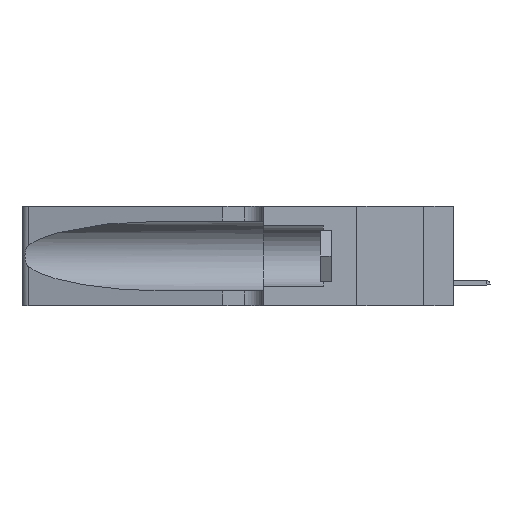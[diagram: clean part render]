
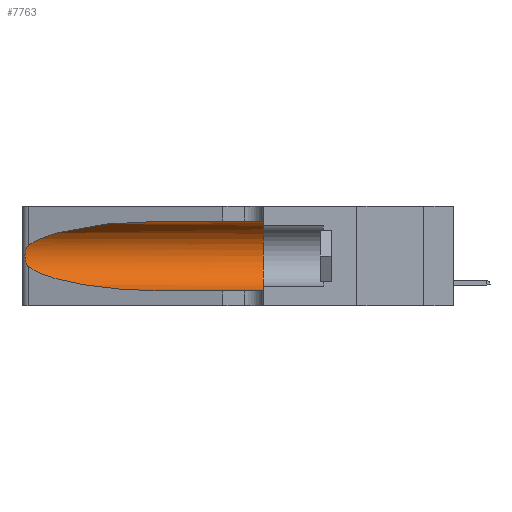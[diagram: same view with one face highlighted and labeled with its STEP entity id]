
A CAD part, left-side view. The second image highlights one B-rep face of the part: STEP entity #7763.
In plain terms, the highlighted cylindrical face has radius 3.308 mm (diameter 6.617 mm), a partial arc.
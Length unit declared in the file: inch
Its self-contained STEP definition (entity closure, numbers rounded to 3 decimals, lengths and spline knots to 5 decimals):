
#553 = CARTESIAN_POINT ( 'NONE',  ( 0.2373, 1.15595, 0.08982 ) ) ;
#1433 = VERTEX_POINT ( 'NONE', #5985 ) ;
#1889 = LINE ( 'NONE', #8013, #12411 ) ;
#2998 = CARTESIAN_POINT ( 'NONE',  ( 0.1305, 1.61858, 0.185 ) ) ;
#3121 = EDGE_CURVE ( 'NONE', #13543, #18669, #11058, .T. ) ;
#3147 = AXIS2_PLACEMENT_3D ( 'NONE', #6868, #18050, #10074 ) ;
#3162 = ORIENTED_EDGE ( 'NONE', *, *, #3121, .T. ) ;
#3216 = DIRECTION ( 'NONE',  ( 0., 0., -1. ) ) ;
#3707 = VERTEX_POINT ( 'NONE', #13667 ) ;
#4069 = CARTESIAN_POINT ( 'NONE',  ( 0.25854, 1.2359, 0.20912 ) ) ;
#5098 = B_SPLINE_CURVE_WITH_KNOTS ( 'NONE', 3,
 ( #20478, #20588, #10875, #18629, #4069, #10568, #12259, #18740, #16200, #16524, #8134, #11315, #17808, #18129 ),
 .UNSPECIFIED., .F., .F.,
 ( 4, 2, 2, 2, 2, 2, 4 ),
 ( 0., 0.00027, 0.00053, 0.00107, 0.0016, 0.00187, 0.00214 ),
 .UNSPECIFIED. ) ;
#5554 = CARTESIAN_POINT ( 'NONE',  ( 0.2373, 1.15595, 0.28018 ) ) ;
#5985 = CARTESIAN_POINT ( 'NONE',  ( 0.1305, 0.72297, 0.05475 ) ) ;
#6702 =( BOUNDED_CURVE ( )  B_SPLINE_CURVE ( 3, ( #13577, #553, #7199, #13686 ),
 .UNSPECIFIED., .F., .T. ) 
 B_SPLINE_CURVE_WITH_KNOTS ( ( 4, 4 ),
 ( 3.44316, 4.71239 ),
 .UNSPECIFIED. ) 
 CURVE ( )  GEOMETRIC_REPRESENTATION_ITEM ( )  RATIONAL_B_SPLINE_CURVE ( ( 1., 0.87, 0.87, 1. ) ) 
 REPRESENTATION_ITEM ( '' )  );
#6868 = CARTESIAN_POINT ( 'NONE',  ( 0.1305, 0.35, 0.185 ) ) ;
#7199 = CARTESIAN_POINT ( 'NONE',  ( 0.18966, 0.96281, 0.05475 ) ) ;
#7763 = ADVANCED_FACE ( 'NONE', ( #19625 ), #21017, .F. ) ;
#7794 = CARTESIAN_POINT ( 'NONE',  ( 0.1305, 1.61858, 0.31525 ) ) ;
#8013 = CARTESIAN_POINT ( 'NONE',  ( 0.1305, 1.61858, 0.05475 ) ) ;
#8134 = CARTESIAN_POINT ( 'NONE',  ( 0.25789, 1.23486, 0.15765 ) ) ;
#8591 = CARTESIAN_POINT ( 'NONE',  ( 0.1305, 0.35, 0.05475 ) ) ;
#9080 = EDGE_CURVE ( 'NONE', #18669, #17951, #5098, .T. ) ;
#9188 = CARTESIAN_POINT ( 'NONE',  ( 0.1305, 0.72297, 0.31525 ) ) ;
#10074 = DIRECTION ( 'NONE',  ( 0., 0., 1. ) ) ;
#10568 = CARTESIAN_POINT ( 'NONE',  ( 0.26018, 1.23835, 0.19895 ) ) ;
#10875 = CARTESIAN_POINT ( 'NONE',  ( 0.25639, 1.23184, 0.21858 ) ) ;
#11058 =( BOUNDED_CURVE ( )  B_SPLINE_CURVE ( 3, ( #15146, #20172, #5554, #12067 ),
 .UNSPECIFIED., .F., .T. ) 
 B_SPLINE_CURVE_WITH_KNOTS ( ( 4, 4 ),
 ( 1.5708, 2.84003 ),
 .UNSPECIFIED. ) 
 CURVE ( )  GEOMETRIC_REPRESENTATION_ITEM ( )  RATIONAL_B_SPLINE_CURVE ( ( 1., 0.87, 0.87, 1. ) ) 
 REPRESENTATION_ITEM ( '' )  );
#11315 = CARTESIAN_POINT ( 'NONE',  ( 0.25639, 1.23186, 0.15144 ) ) ;
#12067 = CARTESIAN_POINT ( 'NONE',  ( 0.25487, 1.22718, 0.22369 ) ) ;
#12256 = VECTOR ( 'NONE', #14303, 39.37008 ) ;
#12259 = CARTESIAN_POINT ( 'NONE',  ( 0.26075, 1.23896, 0.19203 ) ) ;
#12411 = VECTOR ( 'NONE', #16303, 39.37008 ) ;
#12804 = DIRECTION ( 'NONE',  ( 0., -1., 0. ) ) ;
#12899 = EDGE_CURVE ( 'NONE', #1433, #13908, #1889, .T. ) ;
#12971 = ORIENTED_EDGE ( 'NONE', *, *, #17817, .T. ) ;
#13543 = VERTEX_POINT ( 'NONE', #9188 ) ;
#13577 = CARTESIAN_POINT ( 'NONE',  ( 0.25487, 1.22718, 0.14631 ) ) ;
#13667 = CARTESIAN_POINT ( 'NONE',  ( 0.1305, 0.35, 0.31525 ) ) ;
#13686 = CARTESIAN_POINT ( 'NONE',  ( 0.1305, 0.72297, 0.05475 ) ) ;
#13908 = VERTEX_POINT ( 'NONE', #8591 ) ;
#14303 = DIRECTION ( 'NONE',  ( 0., -1., 0. ) ) ;
#14854 = ORIENTED_EDGE ( 'NONE', *, *, #18450, .F. ) ;
#15041 = ORIENTED_EDGE ( 'NONE', *, *, #9080, .T. ) ;
#15146 = CARTESIAN_POINT ( 'NONE',  ( 0.1305, 0.72297, 0.31525 ) ) ;
#15693 = CARTESIAN_POINT ( 'NONE',  ( 0.25487, 1.22718, 0.14631 ) ) ;
#15721 = CIRCLE ( 'NONE', #3147, 0.13025 ) ;
#15977 = LINE ( 'NONE', #7794, #12256 ) ;
#16200 = CARTESIAN_POINT ( 'NONE',  ( 0.26017, 1.23833, 0.17102 ) ) ;
#16303 = DIRECTION ( 'NONE',  ( 0., -1., 0. ) ) ;
#16524 = CARTESIAN_POINT ( 'NONE',  ( 0.25856, 1.23593, 0.16098 ) ) ;
#16730 = EDGE_LOOP ( 'NONE', ( #3162, #15041, #12971, #20121, #20022, #14854 ) ) ;
#16893 = AXIS2_PLACEMENT_3D ( 'NONE', #2998, #12804, #3216 ) ;
#17808 = CARTESIAN_POINT ( 'NONE',  ( 0.25555, 1.22993, 0.14849 ) ) ;
#17817 = EDGE_CURVE ( 'NONE', #17951, #1433, #6702, .T. ) ;
#17951 = VERTEX_POINT ( 'NONE', #15693 ) ;
#18050 = DIRECTION ( 'NONE',  ( 0., 1., 0. ) ) ;
#18129 = CARTESIAN_POINT ( 'NONE',  ( 0.25487, 1.22718, 0.14631 ) ) ;
#18450 = EDGE_CURVE ( 'NONE', #13543, #3707, #15977, .T. ) ;
#18494 = CARTESIAN_POINT ( 'NONE',  ( 0.25487, 1.22718, 0.22369 ) ) ;
#18629 = CARTESIAN_POINT ( 'NONE',  ( 0.25787, 1.23484, 0.2124 ) ) ;
#18669 = VERTEX_POINT ( 'NONE', #18494 ) ;
#18740 = CARTESIAN_POINT ( 'NONE',  ( 0.26075, 1.23896, 0.178 ) ) ;
#19625 = FACE_OUTER_BOUND ( 'NONE', #16730, .T. ) ;
#20022 = ORIENTED_EDGE ( 'NONE', *, *, #20466, .F. ) ;
#20121 = ORIENTED_EDGE ( 'NONE', *, *, #12899, .T. ) ;
#20172 = CARTESIAN_POINT ( 'NONE',  ( 0.18966, 0.96281, 0.31525 ) ) ;
#20466 = EDGE_CURVE ( 'NONE', #3707, #13908, #15721, .T. ) ;
#20478 = CARTESIAN_POINT ( 'NONE',  ( 0.25487, 1.22718, 0.22369 ) ) ;
#20588 = CARTESIAN_POINT ( 'NONE',  ( 0.25555, 1.22994, 0.2215 ) ) ;
#21017 = CYLINDRICAL_SURFACE ( 'NONE', #16893, 0.13025 ) ;
